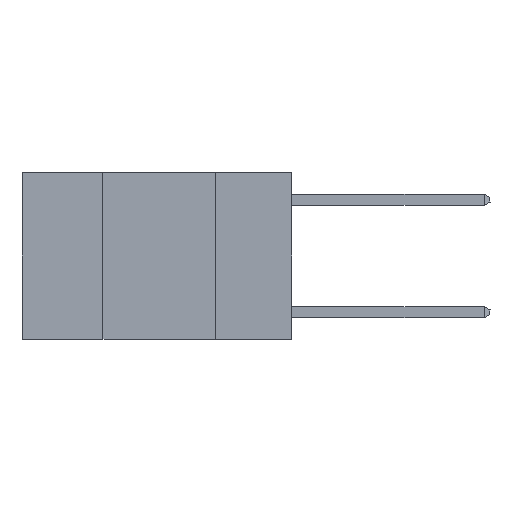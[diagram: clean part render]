
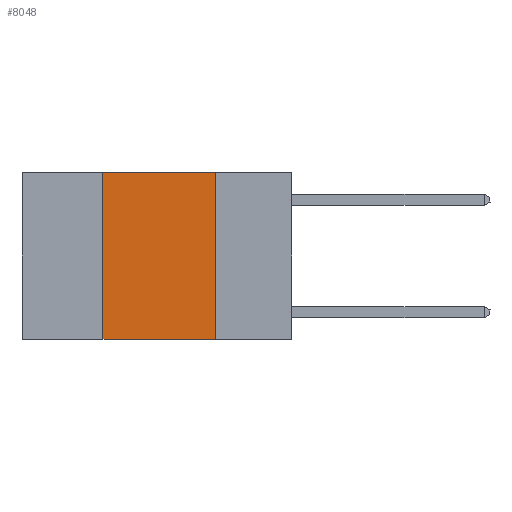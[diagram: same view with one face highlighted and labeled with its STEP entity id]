
A CAD part, left-side view. The second image highlights one B-rep face of the part: STEP entity #8048.
In plain terms, the highlighted planar face has unit normal (-1, 0, 0).
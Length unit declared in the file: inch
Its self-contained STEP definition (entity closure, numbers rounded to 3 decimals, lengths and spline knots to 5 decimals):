
#148 = VERTEX_POINT ( 'NONE', #15479 ) ;
#446 = DIRECTION ( 'NONE',  ( 0., 0., -1. ) ) ;
#611 = CARTESIAN_POINT ( 'NONE',  ( 0., 0.6, -0.37 ) ) ;
#622 = VERTEX_POINT ( 'NONE', #14247 ) ;
#932 = EDGE_CURVE ( 'NONE', #3537, #622, #10924, .T. ) ;
#972 = ORIENTED_EDGE ( 'NONE', *, *, #8958, .F. ) ;
#997 = DIRECTION ( 'NONE',  ( 0., -1., 0. ) ) ;
#1289 = VECTOR ( 'NONE', #8682, 39.37008 ) ;
#3537 = VERTEX_POINT ( 'NONE', #4281 ) ;
#3997 = DIRECTION ( 'NONE',  ( 0., -1., 0. ) ) ;
#4153 = CARTESIAN_POINT ( 'NONE',  ( 0., 0.42, 0. ) ) ;
#4281 = CARTESIAN_POINT ( 'NONE',  ( 0., 0.42, -0.37 ) ) ;
#4704 = DIRECTION ( 'NONE',  ( 0., 0., 1. ) ) ;
#5374 = VECTOR ( 'NONE', #3997, 39.37008 ) ;
#5975 = CARTESIAN_POINT ( 'NONE',  ( 0., 0.42, 0. ) ) ;
#6503 = EDGE_LOOP ( 'NONE', ( #13147, #7796, #972, #12386 ) ) ;
#6611 = EDGE_CURVE ( 'NONE', #148, #622, #14225, .T. ) ;
#6842 = PLANE ( 'NONE',  #10587 ) ;
#7423 = VERTEX_POINT ( 'NONE', #4153 ) ;
#7647 = VECTOR ( 'NONE', #997, 39.37008 ) ;
#7796 = ORIENTED_EDGE ( 'NONE', *, *, #15037, .F. ) ;
#8048 = ADVANCED_FACE ( 'NONE', ( #16090 ), #6842, .F. ) ;
#8116 = DIRECTION ( 'NONE',  ( 1., 0., 0. ) ) ;
#8682 = DIRECTION ( 'NONE',  ( 0., 0., -1. ) ) ;
#8958 = EDGE_CURVE ( 'NONE', #3537, #7423, #9207, .T. ) ;
#9207 = LINE ( 'NONE', #5975, #15299 ) ;
#10587 = AXIS2_PLACEMENT_3D ( 'NONE', #15422, #8116, #446 ) ;
#10924 = LINE ( 'NONE', #611, #7647 ) ;
#11458 = CARTESIAN_POINT ( 'NONE',  ( 0., 0.6, 0. ) ) ;
#12386 = ORIENTED_EDGE ( 'NONE', *, *, #932, .T. ) ;
#13147 = ORIENTED_EDGE ( 'NONE', *, *, #6611, .F. ) ;
#14225 = LINE ( 'NONE', #15963, #1289 ) ;
#14247 = CARTESIAN_POINT ( 'NONE',  ( 0., 0.17, -0.37 ) ) ;
#14846 = LINE ( 'NONE', #11458, #5374 ) ;
#15037 = EDGE_CURVE ( 'NONE', #7423, #148, #14846, .T. ) ;
#15299 = VECTOR ( 'NONE', #4704, 39.37008 ) ;
#15422 = CARTESIAN_POINT ( 'NONE',  ( 0., 0.6, 0. ) ) ;
#15479 = CARTESIAN_POINT ( 'NONE',  ( 0., 0.17, 0. ) ) ;
#15963 = CARTESIAN_POINT ( 'NONE',  ( 0., 0.17, 0. ) ) ;
#16090 = FACE_OUTER_BOUND ( 'NONE', #6503, .T. ) ;
